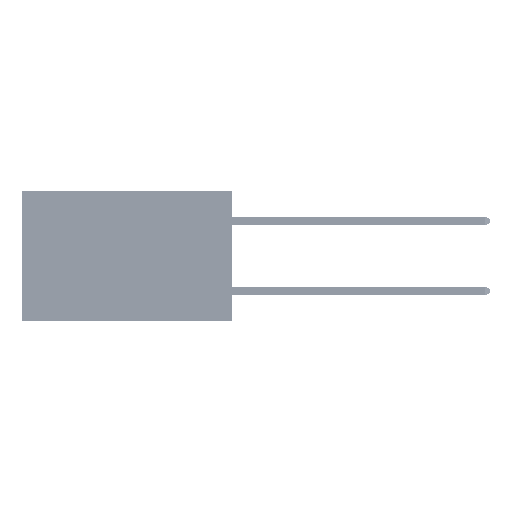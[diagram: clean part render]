
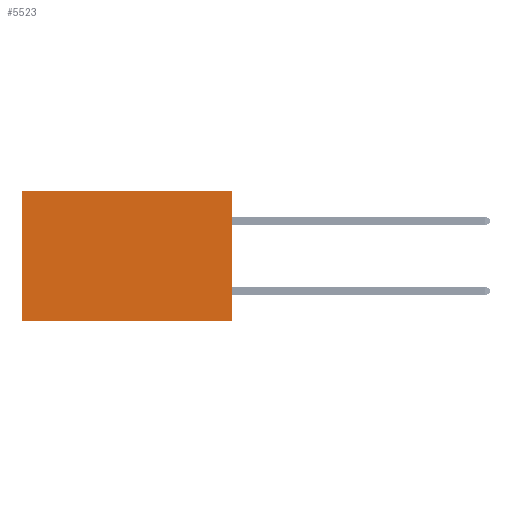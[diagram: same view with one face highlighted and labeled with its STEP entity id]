
A CAD part, left-side view. The second image highlights one B-rep face of the part: STEP entity #5523.
In plain terms, the highlighted planar face has unit normal (-1, 0, 0).
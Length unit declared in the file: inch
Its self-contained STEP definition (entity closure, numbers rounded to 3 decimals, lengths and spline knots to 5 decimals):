
#852 = EDGE_CURVE ( 'NONE', #29657, #46060, #41451, .T. ) ;
#1452 = CARTESIAN_POINT ( 'NONE',  ( 0.2875, 0., 0. ) ) ;
#2362 = VERTEX_POINT ( 'NONE', #5964 ) ;
#3279 = CARTESIAN_POINT ( 'NONE',  ( 0.2875, 0., 0. ) ) ;
#3670 = LINE ( 'NONE', #3279, #45655 ) ;
#4871 = DIRECTION ( 'NONE',  ( 0., 0., -1. ) ) ;
#5449 = ORIENTED_EDGE ( 'NONE', *, *, #19520, .F. ) ;
#5487 = LINE ( 'NONE', #39505, #40626 ) ;
#5523 = ADVANCED_FACE ( 'NONE', ( #9502 ), #35473, .F. ) ;
#5847 = CARTESIAN_POINT ( 'NONE',  ( 0.2875, 0., -0.37 ) ) ;
#5964 = CARTESIAN_POINT ( 'NONE',  ( 0.2875, 0.6, 0. ) ) ;
#9502 = FACE_OUTER_BOUND ( 'NONE', #36449, .T. ) ;
#13755 = ORIENTED_EDGE ( 'NONE', *, *, #852, .F. ) ;
#15280 = CARTESIAN_POINT ( 'NONE',  ( 0.2875, 0., 0. ) ) ;
#17060 = DIRECTION ( 'NONE',  ( 0., 0., -1. ) ) ;
#18167 = CARTESIAN_POINT ( 'NONE',  ( 0.2875, 0.6, -0.37 ) ) ;
#18185 = VECTOR ( 'NONE', #4871, 39.37008 ) ;
#19520 = EDGE_CURVE ( 'NONE', #43849, #29657, #34376, .T. ) ;
#20801 = DIRECTION ( 'NONE',  ( 0., 0., -1. ) ) ;
#23033 = VECTOR ( 'NONE', #32384, 39.37008 ) ;
#27434 = DIRECTION ( 'NONE',  ( 1., 0., 0. ) ) ;
#29657 = VERTEX_POINT ( 'NONE', #5847 ) ;
#31731 = ORIENTED_EDGE ( 'NONE', *, *, #41457, .T. ) ;
#31773 = AXIS2_PLACEMENT_3D ( 'NONE', #38543, #27434, #17060 ) ;
#32384 = DIRECTION ( 'NONE',  ( 0., 1., 0. ) ) ;
#34376 = LINE ( 'NONE', #15280, #18185 ) ;
#34714 = ORIENTED_EDGE ( 'NONE', *, *, #42292, .T. ) ;
#35473 = PLANE ( 'NONE',  #31773 ) ;
#36449 = EDGE_LOOP ( 'NONE', ( #31731, #13755, #5449, #34714 ) ) ;
#38543 = CARTESIAN_POINT ( 'NONE',  ( 0.2875, 0., 0. ) ) ;
#39505 = CARTESIAN_POINT ( 'NONE',  ( 0.2875, 0.6, 0. ) ) ;
#39780 = CARTESIAN_POINT ( 'NONE',  ( 0.2875, 0., -0.37 ) ) ;
#40626 = VECTOR ( 'NONE', #20801, 39.37008 ) ;
#41451 = LINE ( 'NONE', #39780, #23033 ) ;
#41457 = EDGE_CURVE ( 'NONE', #2362, #46060, #5487, .T. ) ;
#42292 = EDGE_CURVE ( 'NONE', #43849, #2362, #3670, .T. ) ;
#43849 = VERTEX_POINT ( 'NONE', #1452 ) ;
#45655 = VECTOR ( 'NONE', #46874, 39.37008 ) ;
#46060 = VERTEX_POINT ( 'NONE', #18167 ) ;
#46874 = DIRECTION ( 'NONE',  ( 0., 1., 0. ) ) ;
